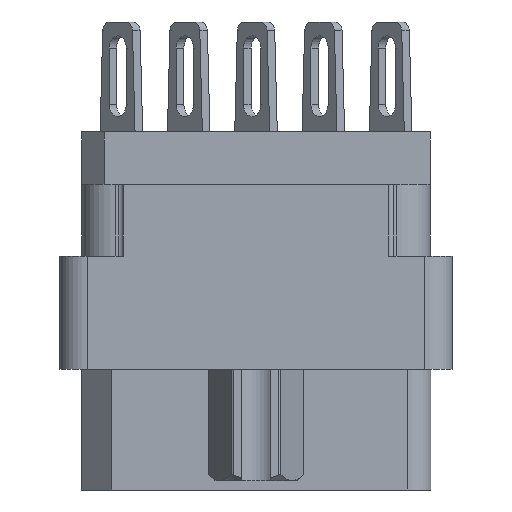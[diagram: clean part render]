
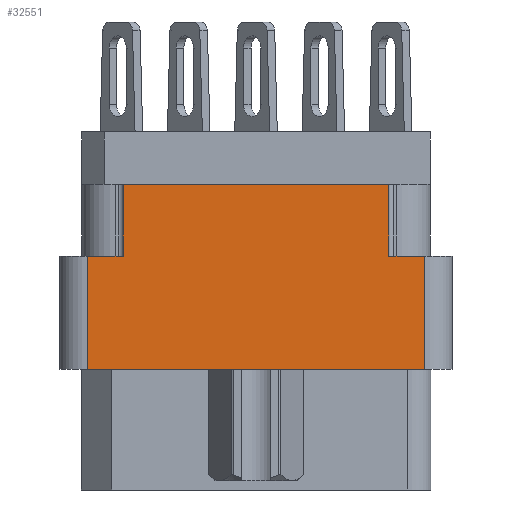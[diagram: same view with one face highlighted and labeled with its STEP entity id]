
A CAD part, left-side view. The second image highlights one B-rep face of the part: STEP entity #32551.
In plain terms, the highlighted planar face has unit normal (-1, 0, 0).
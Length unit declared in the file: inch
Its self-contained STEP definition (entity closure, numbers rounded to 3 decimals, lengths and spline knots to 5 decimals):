
#343 = CARTESIAN_POINT ( 'NONE',  ( -1., -0.296, -0.277 ) ) ;
#694 = CARTESIAN_POINT ( 'NONE',  ( -1., -0.296, -0.277 ) ) ;
#998 = VERTEX_POINT ( 'NONE', #11899 ) ;
#1451 = ORIENTED_EDGE ( 'NONE', *, *, #28159, .F. ) ;
#2054 = FACE_OUTER_BOUND ( 'NONE', #44634, .T. ) ;
#3149 = LINE ( 'NONE', #45217, #31128 ) ;
#4559 = LINE ( 'NONE', #7969, #16733 ) ;
#4862 = VECTOR ( 'NONE', #37840, 39.37008 ) ;
#5303 = CARTESIAN_POINT ( 'NONE',  ( -1., -0.296, -0.277 ) ) ;
#5386 = LINE ( 'NONE', #19333, #11364 ) ;
#5543 = VECTOR ( 'NONE', #27518, 39.37008 ) ;
#6538 = EDGE_CURVE ( 'NONE', #39999, #33804, #4559, .T. ) ;
#6635 = VERTEX_POINT ( 'NONE', #37241 ) ;
#6699 = DIRECTION ( 'NONE',  ( 0., -1., 0. ) ) ;
#7603 = ORIENTED_EDGE ( 'NONE', *, *, #41353, .T. ) ;
#7969 = CARTESIAN_POINT ( 'NONE',  ( -1., 0.296, -0.277 ) ) ;
#9963 = DIRECTION ( 'NONE',  ( 0., 0., 1. ) ) ;
#10345 = LINE ( 'NONE', #31644, #5543 ) ;
#10513 = EDGE_CURVE ( 'NONE', #36602, #39999, #44683, .T. ) ;
#10517 = VERTEX_POINT ( 'NONE', #37578 ) ;
#11364 = VECTOR ( 'NONE', #23675, 39.37008 ) ;
#11569 = EDGE_CURVE ( 'NONE', #24648, #6635, #27793, .T. ) ;
#11899 = CARTESIAN_POINT ( 'NONE',  ( -1., -0.296, -0.117 ) ) ;
#12752 = EDGE_CURVE ( 'NONE', #31969, #6635, #3149, .T. ) ;
#13230 = PLANE ( 'NONE',  #28437 ) ;
#14251 = DIRECTION ( 'NONE',  ( 0., -1., 0. ) ) ;
#14382 = CARTESIAN_POINT ( 'NONE',  ( -1., 0.296, -0.277 ) ) ;
#16660 = DIRECTION ( 'NONE',  ( -1., 0., 0. ) ) ;
#16714 = ORIENTED_EDGE ( 'NONE', *, *, #12752, .T. ) ;
#16733 = VECTOR ( 'NONE', #32483, 39.37008 ) ;
#17507 = ORIENTED_EDGE ( 'NONE', *, *, #10513, .F. ) ;
#19333 = CARTESIAN_POINT ( 'NONE',  ( -1., 0.376, -0.798 ) ) ;
#23675 = DIRECTION ( 'NONE',  ( 0., 0., 1. ) ) ;
#24648 = VERTEX_POINT ( 'NONE', #5303 ) ;
#25152 = LINE ( 'NONE', #694, #32557 ) ;
#25463 = CARTESIAN_POINT ( 'NONE',  ( -1., 0.296, -0.117 ) ) ;
#27121 = LINE ( 'NONE', #41063, #4862 ) ;
#27209 = CARTESIAN_POINT ( 'NONE',  ( -1., -0.376, -0.798 ) ) ;
#27495 = VECTOR ( 'NONE', #14251, 39.37008 ) ;
#27518 = DIRECTION ( 'NONE',  ( 0., 1., 0. ) ) ;
#27771 = CARTESIAN_POINT ( 'NONE',  ( -1., 0.438, -0.277 ) ) ;
#27793 = LINE ( 'NONE', #343, #27495 ) ;
#28159 = EDGE_CURVE ( 'NONE', #10517, #36602, #5386, .T. ) ;
#28177 = CARTESIAN_POINT ( 'NONE',  ( -1., 0.376, -0.277 ) ) ;
#28327 = CARTESIAN_POINT ( 'NONE',  ( -1., -0.376, -0.529 ) ) ;
#28437 = AXIS2_PLACEMENT_3D ( 'NONE', #27209, #16660, #40465 ) ;
#29281 = EDGE_CURVE ( 'NONE', #33804, #998, #27121, .T. ) ;
#29624 = VECTOR ( 'NONE', #6699, 39.37008 ) ;
#30564 = ORIENTED_EDGE ( 'NONE', *, *, #11569, .F. ) ;
#31128 = VECTOR ( 'NONE', #9963, 39.37008 ) ;
#31644 = CARTESIAN_POINT ( 'NONE',  ( -1., -0.376, -0.529 ) ) ;
#31969 = VERTEX_POINT ( 'NONE', #28327 ) ;
#32483 = DIRECTION ( 'NONE',  ( 0., 0., 1. ) ) ;
#32551 = ADVANCED_FACE ( 'NONE', ( #2054 ), #13230, .T. ) ;
#32557 = VECTOR ( 'NONE', #39084, 39.37008 ) ;
#33804 = VERTEX_POINT ( 'NONE', #25463 ) ;
#36602 = VERTEX_POINT ( 'NONE', #28177 ) ;
#36970 = ORIENTED_EDGE ( 'NONE', *, *, #40694, .F. ) ;
#37241 = CARTESIAN_POINT ( 'NONE',  ( -1., -0.376, -0.277 ) ) ;
#37578 = CARTESIAN_POINT ( 'NONE',  ( -1., 0.376, -0.529 ) ) ;
#37840 = DIRECTION ( 'NONE',  ( 0., -1., 0. ) ) ;
#39084 = DIRECTION ( 'NONE',  ( 0., 0., 1. ) ) ;
#39999 = VERTEX_POINT ( 'NONE', #14382 ) ;
#40064 = ORIENTED_EDGE ( 'NONE', *, *, #6538, .F. ) ;
#40465 = DIRECTION ( 'NONE',  ( 0., 0., 1. ) ) ;
#40694 = EDGE_CURVE ( 'NONE', #31969, #10517, #10345, .T. ) ;
#41063 = CARTESIAN_POINT ( 'NONE',  ( -1., 0.438, -0.117 ) ) ;
#41353 = EDGE_CURVE ( 'NONE', #24648, #998, #25152, .T. ) ;
#44220 = ORIENTED_EDGE ( 'NONE', *, *, #29281, .F. ) ;
#44634 = EDGE_LOOP ( 'NONE', ( #1451, #36970, #16714, #30564, #7603, #44220, #40064, #17507 ) ) ;
#44683 = LINE ( 'NONE', #27771, #29624 ) ;
#45217 = CARTESIAN_POINT ( 'NONE',  ( -1., -0.376, -0.798 ) ) ;
